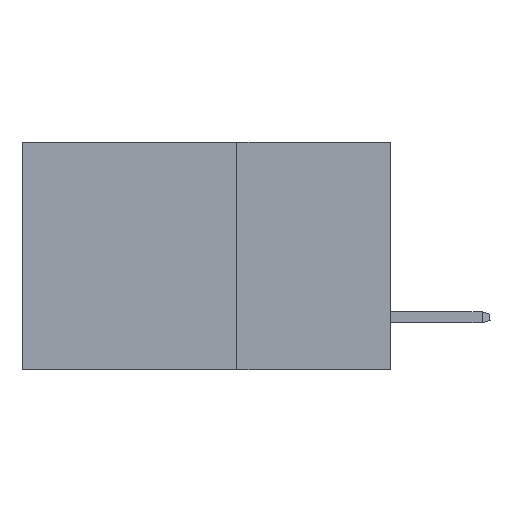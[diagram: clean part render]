
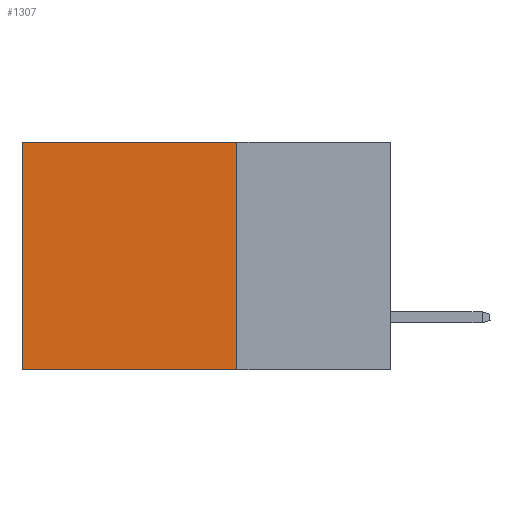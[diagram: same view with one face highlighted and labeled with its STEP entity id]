
A CAD part, left-side view. The second image highlights one B-rep face of the part: STEP entity #1307.
In plain terms, the highlighted planar face has unit normal (-1, 0, 0).
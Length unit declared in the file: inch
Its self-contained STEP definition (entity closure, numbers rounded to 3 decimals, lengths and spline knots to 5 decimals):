
#22 = EDGE_CURVE ( 'NONE', #18592, #2536, #13700, .T. ) ;
#1288 = DIRECTION ( 'NONE',  ( 0., 0., -1. ) ) ;
#1307 = ADVANCED_FACE ( 'NONE', ( #15511 ), #17298, .F. ) ;
#1722 = CARTESIAN_POINT ( 'NONE',  ( 0.2875, 0.6, 0. ) ) ;
#2235 = DIRECTION ( 'NONE',  ( 1., 0., 0. ) ) ;
#2429 = VERTEX_POINT ( 'NONE', #4386 ) ;
#2439 = CARTESIAN_POINT ( 'NONE',  ( 0.2875, 0.25, 0. ) ) ;
#2536 = VERTEX_POINT ( 'NONE', #1722 ) ;
#3628 = DIRECTION ( 'NONE',  ( 0., 1., 0. ) ) ;
#4386 = CARTESIAN_POINT ( 'NONE',  ( 0.2875, 0.25, -0.37 ) ) ;
#5268 = VECTOR ( 'NONE', #1288, 39.37008 ) ;
#5749 = VECTOR ( 'NONE', #18369, 39.37008 ) ;
#6208 = CARTESIAN_POINT ( 'NONE',  ( 0.2875, 0.6, -0.37 ) ) ;
#6430 = VECTOR ( 'NONE', #3628, 39.37008 ) ;
#6525 = CARTESIAN_POINT ( 'NONE',  ( 0.2875, 0.25, 0. ) ) ;
#6626 = CARTESIAN_POINT ( 'NONE',  ( 0.2875, 0.25, -0.37 ) ) ;
#8622 = VERTEX_POINT ( 'NONE', #6208 ) ;
#8922 = ORIENTED_EDGE ( 'NONE', *, *, #18060, .F. ) ;
#10142 = CARTESIAN_POINT ( 'NONE',  ( 0.2875, 0.6, 0. ) ) ;
#10704 = VECTOR ( 'NONE', #18952, 39.37008 ) ;
#11598 = EDGE_CURVE ( 'NONE', #2429, #8622, #17413, .T. ) ;
#11951 = EDGE_CURVE ( 'NONE', #2536, #8622, #14618, .T. ) ;
#12580 = CARTESIAN_POINT ( 'NONE',  ( 0.2875, 0.25, 0. ) ) ;
#12887 = DIRECTION ( 'NONE',  ( 0., 0., -1. ) ) ;
#13029 = EDGE_LOOP ( 'NONE', ( #19115, #13065, #8922, #14583 ) ) ;
#13065 = ORIENTED_EDGE ( 'NONE', *, *, #11598, .F. ) ;
#13464 = AXIS2_PLACEMENT_3D ( 'NONE', #14251, #2235, #12887 ) ;
#13700 = LINE ( 'NONE', #6525, #5749 ) ;
#14251 = CARTESIAN_POINT ( 'NONE',  ( 0.2875, 0.25, 0. ) ) ;
#14583 = ORIENTED_EDGE ( 'NONE', *, *, #22, .T. ) ;
#14618 = LINE ( 'NONE', #10142, #5268 ) ;
#15511 = FACE_OUTER_BOUND ( 'NONE', #13029, .T. ) ;
#17298 = PLANE ( 'NONE',  #13464 ) ;
#17413 = LINE ( 'NONE', #6626, #6430 ) ;
#18060 = EDGE_CURVE ( 'NONE', #18592, #2429, #19118, .T. ) ;
#18369 = DIRECTION ( 'NONE',  ( 0., 1., 0. ) ) ;
#18592 = VERTEX_POINT ( 'NONE', #12580 ) ;
#18952 = DIRECTION ( 'NONE',  ( 0., 0., -1. ) ) ;
#19115 = ORIENTED_EDGE ( 'NONE', *, *, #11951, .T. ) ;
#19118 = LINE ( 'NONE', #2439, #10704 ) ;
